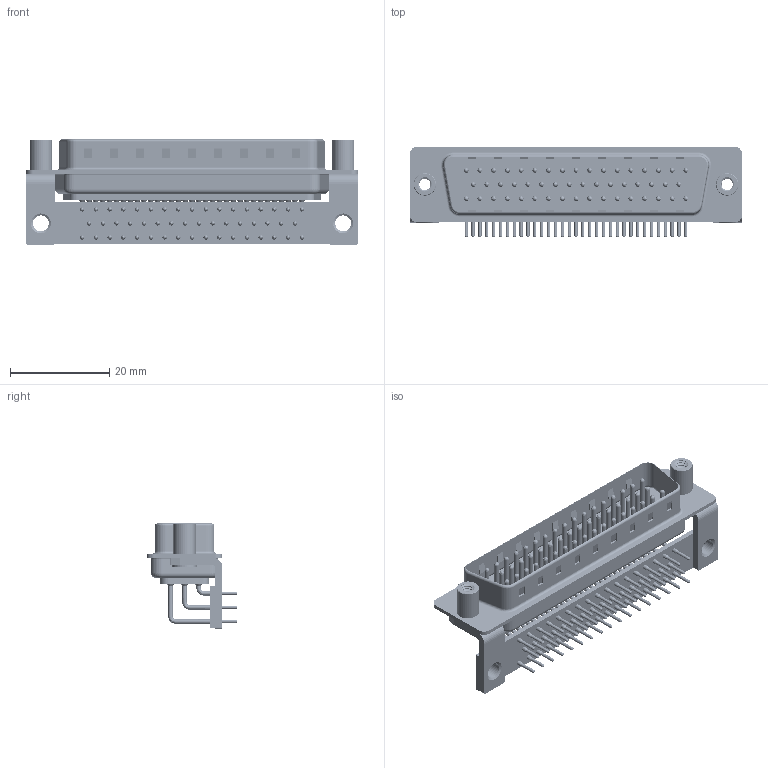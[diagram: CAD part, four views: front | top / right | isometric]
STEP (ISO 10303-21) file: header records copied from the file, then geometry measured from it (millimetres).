
FILE_DESCRIPTION (( 'STEP AP203' ), '1' );
FILE_NAME ('621-M50-260-WN6.STEP', '2018-09-25T11:18:34', ( '' ), ( '' ), 'SwSTEP 2.0', 'SolidWorks 2016', '' );
FILE_SCHEMA (( 'CONFIG_CONTROL_DESIGN' ));
Length unit declared in the file: millimetre
Products named in the file (10): 621-M50-260-WN6; 621M Shell Front_50 Contacts; 621M Shell Rear_50 Contacts; 621M Contact Row 1_50 Contacts; 621M Contact Row 2_50 Contacts; 621M Contact Row 3; 621M Stabilizer Bracket_50 Contacts; 621M 4-40 Threaded Standoff; 621M Stabilizer Board_50 Contacts; 621M Housing_50 Contacts
Assembly tree (58 placements, depth 2):
  621-M50-260-WN6
    621M Housing_50 Contacts
    621M Shell Front_50 Contacts
    621M Shell Rear_50 Contacts
    621M Contact Row 1_50 Contacts  x17
    621M Contact Row 2_50 Contacts  x16
    621M Contact Row 3  x17
    621M Stabilizer Bracket_50 Contacts  x2
    621M 4-40 Threaded Standoff  x2
    621M Stabilizer Board_50 Contacts
Bounding box: 67 x 18.3 x 21.2 mm (x, y, z)
Volume: 5859.7 mm3; surface area: 14876.6 mm2
Topology: 58 solids, 58 shells, 6112 faces, 17161 edges, 11178 vertices
Faces by surface type: plane 3431, cylinder 2105, bspline 306, cone 214, torus 56
Entity records: 43125 total; most frequent: CARTESIAN_POINT 8801, DIRECTION 7031, ORIENTED_EDGE 6378, EDGE_CURVE 3189, AXIS2_PLACEMENT_3D 2643, VERTEX_POINT 2083, LINE 1745, VECTOR 1745
